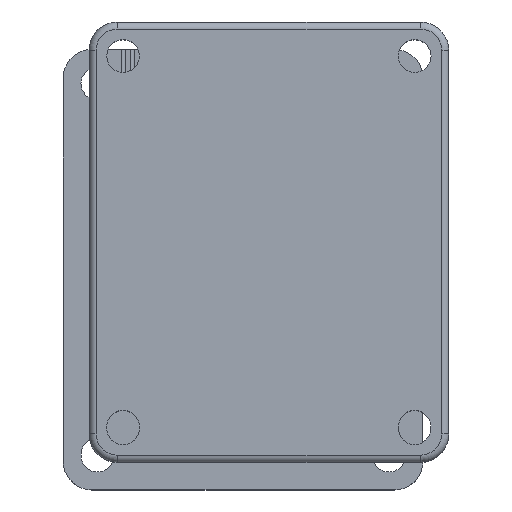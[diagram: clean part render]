
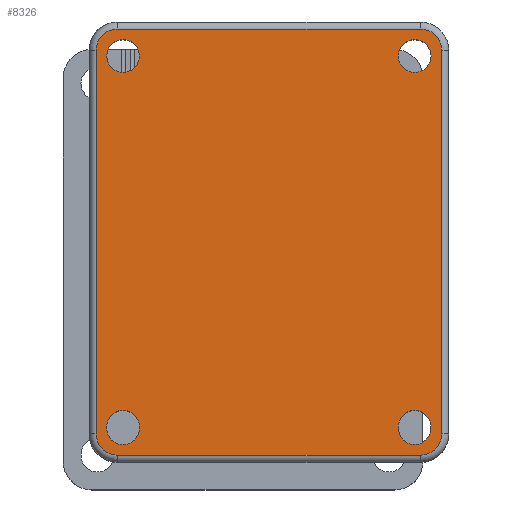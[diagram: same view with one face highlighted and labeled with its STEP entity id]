
A CAD part, top view. The second image highlights one B-rep face of the part: STEP entity #8326.
In plain terms, the highlighted planar face has unit normal (0, 0, 1).
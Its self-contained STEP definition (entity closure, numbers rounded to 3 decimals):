
#492=FACE_BOUND('',#1297,.T.);
#493=FACE_BOUND('',#1298,.T.);
#494=FACE_BOUND('',#1299,.T.);
#495=FACE_BOUND('',#1300,.T.);
#533=PLANE('',#8830);
#818=FACE_OUTER_BOUND('',#1296,.T.);
#1296=EDGE_LOOP('',(#5919,#5920,#5921,#5922,#5923,#5924,#5925,#5926));
#1297=EDGE_LOOP('',(#5927));
#1298=EDGE_LOOP('',(#5928));
#1299=EDGE_LOOP('',(#5929,#5930));
#1300=EDGE_LOOP('',(#5931,#5932));
#1791=LINE('',#10872,#2667);
#1794=LINE('',#10887,#2670);
#1796=LINE('',#10899,#2672);
#1798=LINE('',#10911,#2674);
#2667=VECTOR('',#9200,10.);
#2670=VECTOR('',#9217,10.);
#2672=VECTOR('',#9231,10.);
#2674=VECTOR('',#9245,10.);
#3547=CIRCLE('',#8803,3.);
#3551=CIRCLE('',#8809,3.);
#3555=CIRCLE('',#8815,3.);
#3558=CIRCLE('',#8820,3.);
#3564=CIRCLE('',#8831,2.3);
#3565=CIRCLE('',#8832,2.3);
#3566=CIRCLE('',#8833,2.3);
#3567=CIRCLE('',#8834,2.3);
#3568=CIRCLE('',#8835,2.3);
#3569=CIRCLE('',#8836,2.3);
#3628=VERTEX_POINT('',#10869);
#3629=VERTEX_POINT('',#10871);
#3631=VERTEX_POINT('',#10877);
#3633=VERTEX_POINT('',#10883);
#3635=VERTEX_POINT('',#10889);
#3637=VERTEX_POINT('',#10895);
#3639=VERTEX_POINT('',#10901);
#3641=VERTEX_POINT('',#10907);
#3783=VERTEX_POINT('',#11460);
#3784=VERTEX_POINT('',#11462);
#3785=VERTEX_POINT('',#11464);
#3786=VERTEX_POINT('',#11465);
#3787=VERTEX_POINT('',#11468);
#3788=VERTEX_POINT('',#11469);
#4467=EDGE_CURVE('',#3628,#3629,#1791,.T.);
#4472=EDGE_CURVE('',#3629,#3631,#3547,.T.);
#4475=EDGE_CURVE('',#3631,#3633,#1794,.T.);
#4478=EDGE_CURVE('',#3633,#3635,#3551,.T.);
#4481=EDGE_CURVE('',#3635,#3637,#1796,.T.);
#4484=EDGE_CURVE('',#3637,#3639,#3555,.T.);
#4487=EDGE_CURVE('',#3639,#3641,#1798,.T.);
#4489=EDGE_CURVE('',#3641,#3628,#3558,.T.);
#4634=EDGE_CURVE('',#3783,#3783,#3564,.T.);
#4635=EDGE_CURVE('',#3784,#3784,#3565,.T.);
#4636=EDGE_CURVE('',#3785,#3786,#3566,.T.);
#4637=EDGE_CURVE('',#3786,#3785,#3567,.T.);
#4638=EDGE_CURVE('',#3787,#3788,#3568,.T.);
#4639=EDGE_CURVE('',#3788,#3787,#3569,.T.);
#5919=ORIENTED_EDGE('',*,*,#4467,.F.);
#5920=ORIENTED_EDGE('',*,*,#4489,.F.);
#5921=ORIENTED_EDGE('',*,*,#4487,.F.);
#5922=ORIENTED_EDGE('',*,*,#4484,.F.);
#5923=ORIENTED_EDGE('',*,*,#4481,.F.);
#5924=ORIENTED_EDGE('',*,*,#4478,.F.);
#5925=ORIENTED_EDGE('',*,*,#4475,.F.);
#5926=ORIENTED_EDGE('',*,*,#4472,.F.);
#5927=ORIENTED_EDGE('',*,*,#4634,.T.);
#5928=ORIENTED_EDGE('',*,*,#4635,.T.);
#5929=ORIENTED_EDGE('',*,*,#4636,.T.);
#5930=ORIENTED_EDGE('',*,*,#4637,.T.);
#5931=ORIENTED_EDGE('',*,*,#4638,.T.);
#5932=ORIENTED_EDGE('',*,*,#4639,.T.);
#8326=ADVANCED_FACE('',(#818,#492,#493,#494,#495),#533,.T.);
#8803=AXIS2_PLACEMENT_3D('',#10881,#9210,#9211);
#8809=AXIS2_PLACEMENT_3D('',#10893,#9224,#9225);
#8815=AXIS2_PLACEMENT_3D('',#10905,#9238,#9239);
#8820=AXIS2_PLACEMENT_3D('',#10914,#9250,#9251);
#8830=AXIS2_PLACEMENT_3D('',#11459,#9345,#9346);
#8831=AXIS2_PLACEMENT_3D('',#11461,#9347,#9348);
#8832=AXIS2_PLACEMENT_3D('',#11463,#9349,#9350);
#8833=AXIS2_PLACEMENT_3D('',#11466,#9351,#9352);
#8834=AXIS2_PLACEMENT_3D('',#11467,#9353,#9354);
#8835=AXIS2_PLACEMENT_3D('',#11470,#9355,#9356);
#8836=AXIS2_PLACEMENT_3D('',#11471,#9357,#9358);
#9200=DIRECTION('',(1.,0.,0.));
#9210=DIRECTION('center_axis',(0.,0.,-1.));
#9211=DIRECTION('ref_axis',(0.707,0.707,0.));
#9217=DIRECTION('',(0.,-1.,0.));
#9224=DIRECTION('center_axis',(0.,0.,-1.));
#9225=DIRECTION('ref_axis',(0.707,-0.707,0.));
#9231=DIRECTION('',(-1.,0.,0.));
#9238=DIRECTION('center_axis',(0.,0.,-1.));
#9239=DIRECTION('ref_axis',(-0.707,-0.707,0.));
#9245=DIRECTION('',(0.,1.,0.));
#9250=DIRECTION('center_axis',(0.,0.,-1.));
#9251=DIRECTION('ref_axis',(-0.707,0.707,0.));
#9345=DIRECTION('center_axis',(0.,0.,1.));
#9346=DIRECTION('ref_axis',(1.,0.,0.));
#9347=DIRECTION('center_axis',(0.,0.,-1.));
#9348=DIRECTION('ref_axis',(1.,0.,0.));
#9349=DIRECTION('center_axis',(0.,0.,-1.));
#9350=DIRECTION('ref_axis',(1.,0.,0.));
#9351=DIRECTION('center_axis',(0.,0.,-1.));
#9352=DIRECTION('ref_axis',(1.,0.,0.));
#9353=DIRECTION('center_axis',(0.,0.,-1.));
#9354=DIRECTION('ref_axis',(1.,0.,0.));
#9355=DIRECTION('center_axis',(0.,0.,-1.));
#9356=DIRECTION('ref_axis',(1.,0.,0.));
#9357=DIRECTION('center_axis',(0.,0.,-1.));
#9358=DIRECTION('ref_axis',(1.,0.,0.));
#10869=CARTESIAN_POINT('',(-7.605,109.492,33.292));
#10871=CARTESIAN_POINT('',(35.049,109.492,33.292));
#10872=CARTESIAN_POINT('',(1.058,109.492,33.292));
#10877=CARTESIAN_POINT('',(38.049,106.492,33.292));
#10881=CARTESIAN_POINT('Origin',(35.049,106.492,33.292));
#10883=CARTESIAN_POINT('',(38.049,52.492,33.292));
#10887=CARTESIAN_POINT('',(38.049,3.492,33.292));
#10889=CARTESIAN_POINT('',(35.049,49.492,33.292));
#10893=CARTESIAN_POINT('Origin',(35.049,52.492,33.292));
#10895=CARTESIAN_POINT('',(-7.605,49.492,33.292));
#10899=CARTESIAN_POINT('',(1.058,49.492,33.292));
#10901=CARTESIAN_POINT('',(-10.605,52.492,33.292));
#10905=CARTESIAN_POINT('Origin',(-7.605,52.492,33.292));
#10907=CARTESIAN_POINT('',(-10.605,106.492,33.292));
#10911=CARTESIAN_POINT('',(-10.605,3.492,33.292));
#10914=CARTESIAN_POINT('Origin',(-7.605,106.492,33.292));
#11459=CARTESIAN_POINT('Origin',(-11.605,3.492,33.292));
#11460=CARTESIAN_POINT('',(-9.105,105.692,33.292));
#11461=CARTESIAN_POINT('Origin',(-6.805,105.692,33.292));
#11462=CARTESIAN_POINT('',(31.949,105.692,33.292));
#11463=CARTESIAN_POINT('Origin',(34.249,105.692,33.292));
#11464=CARTESIAN_POINT('',(-4.507,53.392,33.292));
#11465=CARTESIAN_POINT('',(-9.103,53.392,33.292));
#11466=CARTESIAN_POINT('Origin',(-6.805,53.292,33.292));
#11467=CARTESIAN_POINT('Origin',(-6.805,53.492,33.292));
#11468=CARTESIAN_POINT('',(36.547,53.392,33.292));
#11469=CARTESIAN_POINT('',(31.952,53.392,33.292));
#11470=CARTESIAN_POINT('Origin',(34.249,53.292,33.292));
#11471=CARTESIAN_POINT('Origin',(34.249,53.492,33.292));
